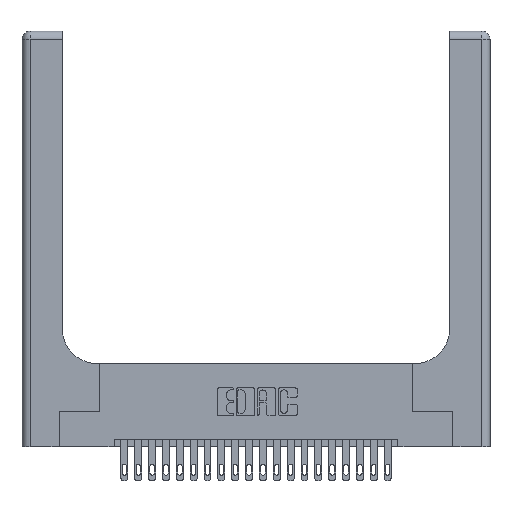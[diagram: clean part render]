
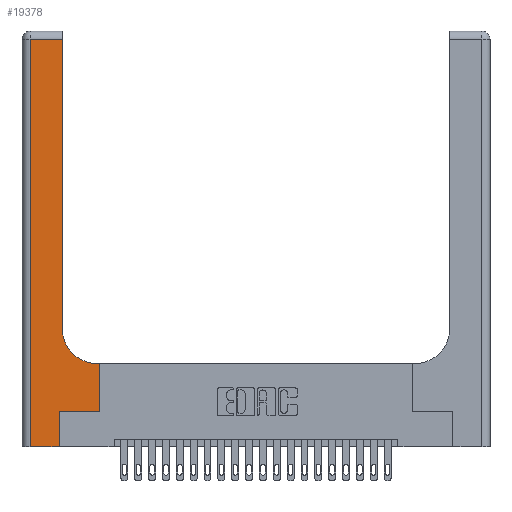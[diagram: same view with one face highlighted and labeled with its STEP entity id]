
A CAD part, top view. The second image highlights one B-rep face of the part: STEP entity #19378.
In plain terms, the highlighted planar face has unit normal (0, 0, 1).
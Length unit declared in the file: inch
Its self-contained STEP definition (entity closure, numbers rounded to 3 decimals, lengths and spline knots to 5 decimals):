
#501 = DIRECTION ( 'NONE',  ( 0., 1., 0. ) ) ;
#563 = ORIENTED_EDGE ( 'NONE', *, *, #5073, .T. ) ;
#741 = CARTESIAN_POINT ( 'NONE',  ( 0.2915, 0.85, 0.37 ) ) ;
#912 = DIRECTION ( 'NONE',  ( 0., 1., 0. ) ) ;
#1005 = DIRECTION ( 'NONE',  ( 0., 0., -1. ) ) ;
#1035 = LINE ( 'NONE', #1517, #18264 ) ;
#1094 = LINE ( 'NONE', #20088, #12533 ) ;
#1115 = VECTOR ( 'NONE', #16720, 39.37008 ) ;
#1166 = CARTESIAN_POINT ( 'NONE',  ( 0.5585, 0.6, 0.37 ) ) ;
#1517 = CARTESIAN_POINT ( 'NONE',  ( 0., 0., 0.37 ) ) ;
#1585 = DIRECTION ( 'NONE',  ( 1., 0., 0. ) ) ;
#2533 = LINE ( 'NONE', #18655, #1115 ) ;
#2910 = VECTOR ( 'NONE', #10669, 39.37008 ) ;
#3376 = CARTESIAN_POINT ( 'NONE',  ( 0.2915, 2.94, 0.37 ) ) ;
#4518 = CARTESIAN_POINT ( 'NONE',  ( 0.06, 2.94, 0.37 ) ) ;
#4776 = VERTEX_POINT ( 'NONE', #4518 ) ;
#5073 = EDGE_CURVE ( 'NONE', #10313, #19501, #9420, .T. ) ;
#5856 = VERTEX_POINT ( 'NONE', #8950 ) ;
#6258 = DIRECTION ( 'NONE',  ( -1., 0., 0. ) ) ;
#7253 = EDGE_CURVE ( 'NONE', #8223, #17941, #1035, .T. ) ;
#7715 = VERTEX_POINT ( 'NONE', #12978 ) ;
#7974 = ORIENTED_EDGE ( 'NONE', *, *, #23200, .T. ) ;
#8126 = CIRCLE ( 'NONE', #8597, 0.25 ) ;
#8223 = VERTEX_POINT ( 'NONE', #21113 ) ;
#8597 = AXIS2_PLACEMENT_3D ( 'NONE', #22158, #20158, #16518 ) ;
#8950 = CARTESIAN_POINT ( 'NONE',  ( 0.5585, 0.25, 0.37 ) ) ;
#9045 = CARTESIAN_POINT ( 'NONE',  ( 0.2915, 0.6, 0.37 ) ) ;
#9199 = ORIENTED_EDGE ( 'NONE', *, *, #17869, .T. ) ;
#9420 = LINE ( 'NONE', #9045, #11734 ) ;
#10012 = CARTESIAN_POINT ( 'NONE',  ( 0.5585, 0.25, 0.37 ) ) ;
#10313 = VERTEX_POINT ( 'NONE', #1166 ) ;
#10484 = ORIENTED_EDGE ( 'NONE', *, *, #7253, .T. ) ;
#10669 = DIRECTION ( 'NONE',  ( 0., -1., 0. ) ) ;
#10787 = LINE ( 'NONE', #15425, #23778 ) ;
#11061 = DIRECTION ( 'NONE',  ( -1., 0., 0. ) ) ;
#11346 = EDGE_CURVE ( 'NONE', #17941, #7715, #19038, .T. ) ;
#11485 = VERTEX_POINT ( 'NONE', #3376 ) ;
#11734 = VECTOR ( 'NONE', #11061, 39.37008 ) ;
#11961 = VERTEX_POINT ( 'NONE', #741 ) ;
#12076 = LINE ( 'NONE', #17994, #2910 ) ;
#12221 = CARTESIAN_POINT ( 'NONE',  ( 0.5415, 0.6, 0.37 ) ) ;
#12338 = ORIENTED_EDGE ( 'NONE', *, *, #12403, .T. ) ;
#12403 = EDGE_CURVE ( 'NONE', #4776, #8223, #12076, .T. ) ;
#12468 = ORIENTED_EDGE ( 'NONE', *, *, #11346, .T. ) ;
#12533 = VECTOR ( 'NONE', #18162, 39.37008 ) ;
#12796 = EDGE_LOOP ( 'NONE', ( #14420, #22373, #12338, #10484, #12468, #14569, #9199, #563, #7974 ) ) ;
#12978 = CARTESIAN_POINT ( 'NONE',  ( 0.269, 0.25, 0.37 ) ) ;
#13194 = LINE ( 'NONE', #10012, #14649 ) ;
#13692 = EDGE_CURVE ( 'NONE', #11961, #11485, #2533, .T. ) ;
#13947 = CARTESIAN_POINT ( 'NONE',  ( 0.269, 0., 0.37 ) ) ;
#14114 = EDGE_CURVE ( 'NONE', #7715, #5856, #1094, .T. ) ;
#14420 = ORIENTED_EDGE ( 'NONE', *, *, #13692, .T. ) ;
#14569 = ORIENTED_EDGE ( 'NONE', *, *, #14114, .T. ) ;
#14649 = VECTOR ( 'NONE', #912, 39.37008 ) ;
#15191 = EDGE_CURVE ( 'NONE', #11485, #4776, #10787, .T. ) ;
#15425 = CARTESIAN_POINT ( 'NONE',  ( 0., 2.94, 0.37 ) ) ;
#15440 = CARTESIAN_POINT ( 'NONE',  ( 0., 3., 0.37 ) ) ;
#16518 = DIRECTION ( 'NONE',  ( 1., 0., 0. ) ) ;
#16720 = DIRECTION ( 'NONE',  ( 0., 1., 0. ) ) ;
#17869 = EDGE_CURVE ( 'NONE', #5856, #10313, #13194, .T. ) ;
#17941 = VERTEX_POINT ( 'NONE', #13947 ) ;
#17994 = CARTESIAN_POINT ( 'NONE',  ( 0.06, 3., 0.37 ) ) ;
#18162 = DIRECTION ( 'NONE',  ( 1., 0., 0. ) ) ;
#18264 = VECTOR ( 'NONE', #1585, 39.37008 ) ;
#18655 = CARTESIAN_POINT ( 'NONE',  ( 0.2915, 3., 0.37 ) ) ;
#19038 = LINE ( 'NONE', #22509, #19617 ) ;
#19378 = ADVANCED_FACE ( 'NONE', ( #21579 ), #21029, .F. ) ;
#19501 = VERTEX_POINT ( 'NONE', #12221 ) ;
#19617 = VECTOR ( 'NONE', #501, 39.37008 ) ;
#20088 = CARTESIAN_POINT ( 'NONE',  ( 0.269, 0.25, 0.37 ) ) ;
#20158 = DIRECTION ( 'NONE',  ( 0., 0., -1. ) ) ;
#20409 = AXIS2_PLACEMENT_3D ( 'NONE', #15440, #1005, #6258 ) ;
#20846 = DIRECTION ( 'NONE',  ( -1., 0., 0. ) ) ;
#21029 = PLANE ( 'NONE',  #20409 ) ;
#21113 = CARTESIAN_POINT ( 'NONE',  ( 0.06, 0., 0.37 ) ) ;
#21579 = FACE_OUTER_BOUND ( 'NONE', #12796, .T. ) ;
#22158 = CARTESIAN_POINT ( 'NONE',  ( 0.5415, 0.85, 0.37 ) ) ;
#22373 = ORIENTED_EDGE ( 'NONE', *, *, #15191, .T. ) ;
#22509 = CARTESIAN_POINT ( 'NONE',  ( 0.269, 0., 0.37 ) ) ;
#23200 = EDGE_CURVE ( 'NONE', #19501, #11961, #8126, .T. ) ;
#23778 = VECTOR ( 'NONE', #20846, 39.37008 ) ;
